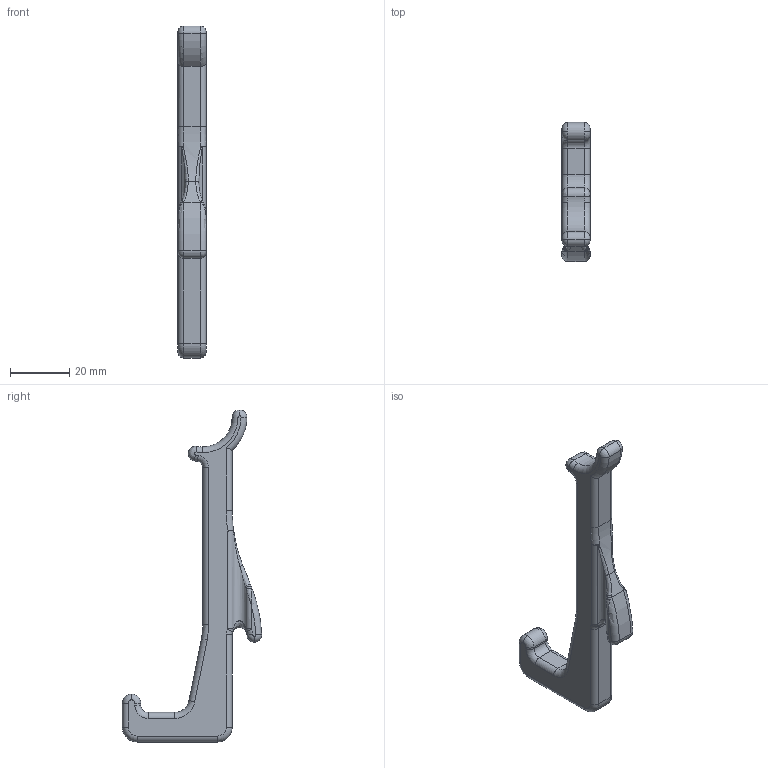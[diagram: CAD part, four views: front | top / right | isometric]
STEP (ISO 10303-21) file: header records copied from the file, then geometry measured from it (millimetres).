
FILE_DESCRIPTION (( 'STEP AP214' ), '1' );
FILE_NAME ('Trigger.STEP', '2013-11-21T02:42:22', ( '' ), ( '' ), 'SwSTEP 2.0', 'SolidWorks 2013', '' );
FILE_SCHEMA (( 'AUTOMOTIVE_DESIGN' ));
Length unit declared in the file: millimetre
Products named in the file (1): Trigger
Bounding box: 9.5 x 47.22 x 112.5 mm (x, y, z)
Volume: 14795.9 mm3; surface area: 5851.6 mm2
Topology: 1 solids, 1 shells, 117 faces, 274 edges, 155 vertices
Faces by surface type: cylinder 41, torus 40, bspline 23, plane 13
Entity records: 4297 total; most frequent: CARTESIAN_POINT 1730, DIRECTION 552, ORIENTED_EDGE 540, EDGE_CURVE 270, AXIS2_PLACEMENT_3D 243, VERTEX_POINT 155, CIRCLE 148, FACE_OUTER_BOUND 117
